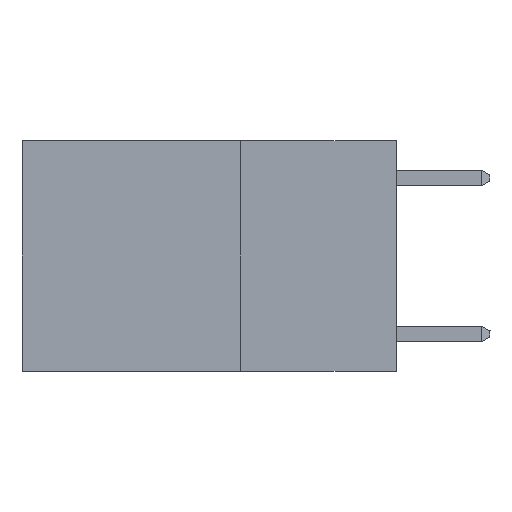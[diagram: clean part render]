
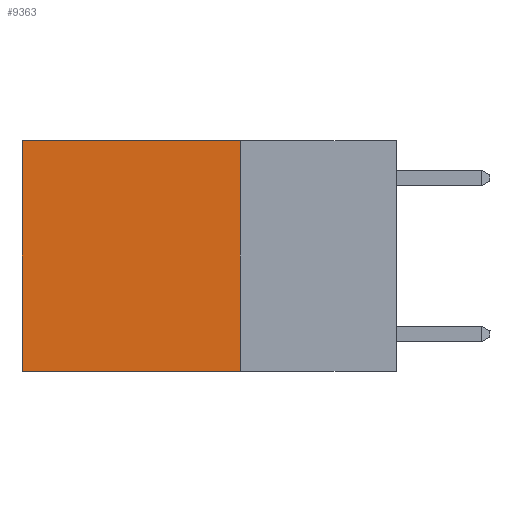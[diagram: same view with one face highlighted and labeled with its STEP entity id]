
A CAD part, left-side view. The second image highlights one B-rep face of the part: STEP entity #9363.
In plain terms, the highlighted planar face has unit normal (-1, 0, 0).
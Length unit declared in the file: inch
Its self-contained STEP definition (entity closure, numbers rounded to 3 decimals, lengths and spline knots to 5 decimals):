
#1950 = CARTESIAN_POINT ( 'NONE',  ( 0.2625, 0.25, -0.37 ) ) ;
#2012 = DIRECTION ( 'NONE',  ( 0., 1., 0. ) ) ;
#3690 = EDGE_LOOP ( 'NONE', ( #6832, #15496, #7608, #5636 ) ) ;
#5162 = DIRECTION ( 'NONE',  ( 1., 0., 0. ) ) ;
#5482 = DIRECTION ( 'NONE',  ( 0., 0., -1. ) ) ;
#5636 = ORIENTED_EDGE ( 'NONE', *, *, #17028, .T. ) ;
#6832 = ORIENTED_EDGE ( 'NONE', *, *, #12761, .T. ) ;
#7226 = CARTESIAN_POINT ( 'NONE',  ( 0.2625, 0.25, 0. ) ) ;
#7247 = VECTOR ( 'NONE', #5482, 39.37008 ) ;
#7608 = ORIENTED_EDGE ( 'NONE', *, *, #10015, .F. ) ;
#8278 = VECTOR ( 'NONE', #10424, 39.37008 ) ;
#8490 = AXIS2_PLACEMENT_3D ( 'NONE', #19483, #5162, #16362 ) ;
#8633 = CARTESIAN_POINT ( 'NONE',  ( 0.2625, 0.25, -0.37 ) ) ;
#8990 = VECTOR ( 'NONE', #2012, 39.37008 ) ;
#9363 = ADVANCED_FACE ( 'NONE', ( #19052 ), #19549, .F. ) ;
#9639 = VERTEX_POINT ( 'NONE', #17394 ) ;
#10015 = EDGE_CURVE ( 'NONE', #20259, #19086, #17274, .T. ) ;
#10424 = DIRECTION ( 'NONE',  ( 0., 1., 0. ) ) ;
#12554 = LINE ( 'NONE', #13941, #8278 ) ;
#12761 = EDGE_CURVE ( 'NONE', #20333, #9639, #14069, .T. ) ;
#13941 = CARTESIAN_POINT ( 'NONE',  ( 0.2625, 0.25, 0. ) ) ;
#14069 = LINE ( 'NONE', #17894, #18074 ) ;
#14473 = CARTESIAN_POINT ( 'NONE',  ( 0.2625, 0.6, 0. ) ) ;
#14515 = EDGE_CURVE ( 'NONE', #19086, #9639, #17492, .T. ) ;
#14609 = DIRECTION ( 'NONE',  ( 0., 0., -1. ) ) ;
#15496 = ORIENTED_EDGE ( 'NONE', *, *, #14515, .F. ) ;
#16362 = DIRECTION ( 'NONE',  ( 0., 0., -1. ) ) ;
#17028 = EDGE_CURVE ( 'NONE', #20259, #20333, #12554, .T. ) ;
#17274 = LINE ( 'NONE', #7226, #7247 ) ;
#17394 = CARTESIAN_POINT ( 'NONE',  ( 0.2625, 0.6, -0.37 ) ) ;
#17492 = LINE ( 'NONE', #1950, #8990 ) ;
#17894 = CARTESIAN_POINT ( 'NONE',  ( 0.2625, 0.6, 0. ) ) ;
#18074 = VECTOR ( 'NONE', #14609, 39.37008 ) ;
#18722 = CARTESIAN_POINT ( 'NONE',  ( 0.2625, 0.25, 0. ) ) ;
#19052 = FACE_OUTER_BOUND ( 'NONE', #3690, .T. ) ;
#19086 = VERTEX_POINT ( 'NONE', #8633 ) ;
#19483 = CARTESIAN_POINT ( 'NONE',  ( 0.2625, 0.25, 0. ) ) ;
#19549 = PLANE ( 'NONE',  #8490 ) ;
#20259 = VERTEX_POINT ( 'NONE', #18722 ) ;
#20333 = VERTEX_POINT ( 'NONE', #14473 ) ;
